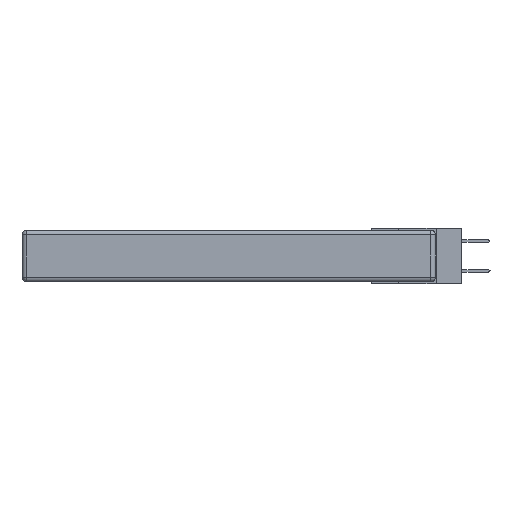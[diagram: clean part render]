
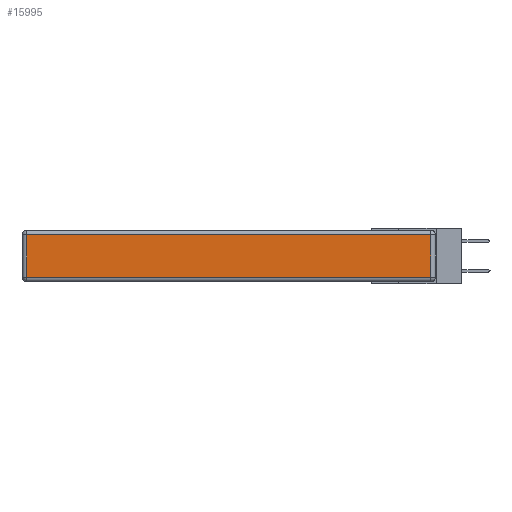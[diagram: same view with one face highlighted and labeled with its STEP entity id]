
A CAD part, left-side view. The second image highlights one B-rep face of the part: STEP entity #15995.
In plain terms, the highlighted planar face has unit normal (-1, 0, 0).
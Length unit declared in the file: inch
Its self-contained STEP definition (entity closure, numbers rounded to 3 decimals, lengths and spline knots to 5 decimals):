
#215 = VECTOR ( 'NONE', #3883, 39.37008 ) ;
#1903 = VERTEX_POINT ( 'NONE', #13522 ) ;
#2261 = CARTESIAN_POINT ( 'NONE',  ( 0., 0., -0.343 ) ) ;
#2302 = EDGE_CURVE ( 'NONE', #8481, #1903, #14218, .T. ) ;
#2578 = FACE_OUTER_BOUND ( 'NONE', #11452, .T. ) ;
#3248 = CARTESIAN_POINT ( 'NONE',  ( 0., 0.03, -0.343 ) ) ;
#3883 = DIRECTION ( 'NONE',  ( 0., 0., -1. ) ) ;
#4975 = DIRECTION ( 'NONE',  ( 0., 0., 1. ) ) ;
#5138 = CARTESIAN_POINT ( 'NONE',  ( 0., 2.72, -0.343 ) ) ;
#5354 = ORIENTED_EDGE ( 'NONE', *, *, #9195, .T. ) ;
#7064 = DIRECTION ( 'NONE',  ( 0., -1., 0. ) ) ;
#7242 = ORIENTED_EDGE ( 'NONE', *, *, #12431, .T. ) ;
#8481 = VERTEX_POINT ( 'NONE', #14106 ) ;
#8622 = CARTESIAN_POINT ( 'NONE',  ( 0., 0., -0.313 ) ) ;
#8625 = VECTOR ( 'NONE', #13944, 39.37008 ) ;
#9195 = EDGE_CURVE ( 'NONE', #15871, #8481, #16673, .T. ) ;
#10699 = DIRECTION ( 'NONE',  ( 0., 1., 0. ) ) ;
#10925 = VERTEX_POINT ( 'NONE', #16851 ) ;
#11452 = EDGE_LOOP ( 'NONE', ( #7242, #5354, #14838, #14806 ) ) ;
#11761 = CARTESIAN_POINT ( 'NONE',  ( 0., 0.03, -0.313 ) ) ;
#12325 = LINE ( 'NONE', #5138, #215 ) ;
#12431 = EDGE_CURVE ( 'NONE', #10925, #15871, #17625, .T. ) ;
#12953 = AXIS2_PLACEMENT_3D ( 'NONE', #2261, #13410, #4975 ) ;
#13410 = DIRECTION ( 'NONE',  ( -1., 0., 0. ) ) ;
#13522 = CARTESIAN_POINT ( 'NONE',  ( 0., 2.72, -0.03 ) ) ;
#13944 = DIRECTION ( 'NONE',  ( 0., 0., 1. ) ) ;
#14106 = CARTESIAN_POINT ( 'NONE',  ( 0., 0.03, -0.03 ) ) ;
#14218 = LINE ( 'NONE', #14731, #14446 ) ;
#14446 = VECTOR ( 'NONE', #10699, 39.37008 ) ;
#14731 = CARTESIAN_POINT ( 'NONE',  ( 0., 2.75, -0.03 ) ) ;
#14806 = ORIENTED_EDGE ( 'NONE', *, *, #15389, .T. ) ;
#14838 = ORIENTED_EDGE ( 'NONE', *, *, #2302, .T. ) ;
#15045 = VECTOR ( 'NONE', #7064, 39.37008 ) ;
#15389 = EDGE_CURVE ( 'NONE', #1903, #10925, #12325, .T. ) ;
#15871 = VERTEX_POINT ( 'NONE', #11761 ) ;
#15995 = ADVANCED_FACE ( 'NONE', ( #2578 ), #16076, .T. ) ;
#16076 = PLANE ( 'NONE',  #12953 ) ;
#16673 = LINE ( 'NONE', #3248, #8625 ) ;
#16851 = CARTESIAN_POINT ( 'NONE',  ( 0., 2.72, -0.313 ) ) ;
#17625 = LINE ( 'NONE', #8622, #15045 ) ;
